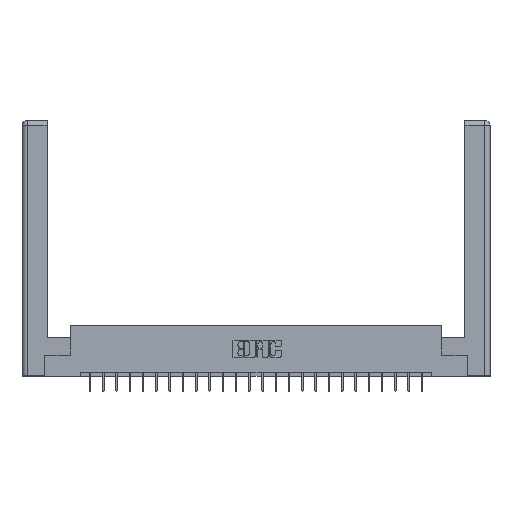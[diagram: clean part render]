
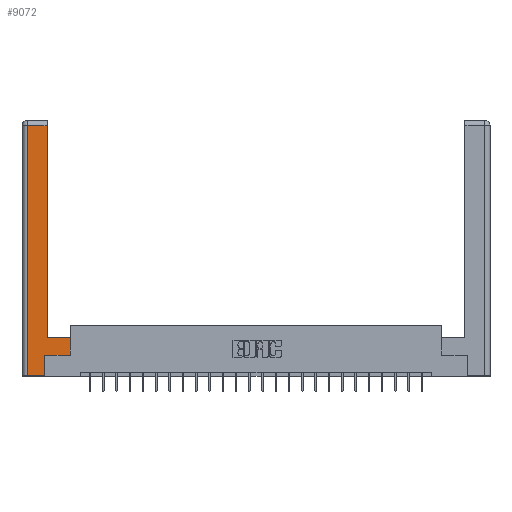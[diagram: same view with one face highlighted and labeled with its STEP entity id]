
A CAD part, top view. The second image highlights one B-rep face of the part: STEP entity #9072.
In plain terms, the highlighted planar face has unit normal (0, 0, 1).
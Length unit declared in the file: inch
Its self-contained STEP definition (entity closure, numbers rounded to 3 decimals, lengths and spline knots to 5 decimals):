
#494 = CARTESIAN_POINT ( 'NONE',  ( 0., 0., 0. ) ) ;
#504 = ORIENTED_EDGE ( 'NONE', *, *, #4105, .T. ) ;
#644 = VERTEX_POINT ( 'NONE', #18237 ) ;
#1146 = CARTESIAN_POINT ( 'NONE',  ( 0.265, 0., 0. ) ) ;
#1230 = VECTOR ( 'NONE', #7607, 39.37008 ) ;
#1911 = VERTEX_POINT ( 'NONE', #3624 ) ;
#1975 = DIRECTION ( 'NONE',  ( 0., 1., 0. ) ) ;
#2231 = CARTESIAN_POINT ( 'NONE',  ( 0.265, 0.245, 0. ) ) ;
#2416 = CARTESIAN_POINT ( 'NONE',  ( 0.295, 2.94, 0. ) ) ;
#2636 = ORIENTED_EDGE ( 'NONE', *, *, #12045, .T. ) ;
#3025 = EDGE_CURVE ( 'NONE', #14537, #15812, #10774, .T. ) ;
#3624 = CARTESIAN_POINT ( 'NONE',  ( 0.565, 0.45, 0. ) ) ;
#4055 = LINE ( 'NONE', #14972, #10418 ) ;
#4105 = EDGE_CURVE ( 'NONE', #8498, #1911, #4055, .T. ) ;
#4262 = ORIENTED_EDGE ( 'NONE', *, *, #11429, .T. ) ;
#4433 = ORIENTED_EDGE ( 'NONE', *, *, #24440, .T. ) ;
#4485 = ORIENTED_EDGE ( 'NONE', *, *, #15095, .T. ) ;
#5100 = CARTESIAN_POINT ( 'NONE',  ( 0.0615, 2.94, 0. ) ) ;
#5492 = AXIS2_PLACEMENT_3D ( 'NONE', #494, #16001, #8128 ) ;
#7195 = EDGE_LOOP ( 'NONE', ( #4262, #15938, #24330, #2636, #11196, #4433, #504, #4485 ) ) ;
#7607 = DIRECTION ( 'NONE',  ( -1., 0., 0. ) ) ;
#7742 = CARTESIAN_POINT ( 'NONE',  ( 0.0615, 2.94, 0. ) ) ;
#7967 = DIRECTION ( 'NONE',  ( -1., 0., 0. ) ) ;
#8015 = VECTOR ( 'NONE', #7967, 39.37008 ) ;
#8128 = DIRECTION ( 'NONE',  ( -1., 0., 0. ) ) ;
#8382 = DIRECTION ( 'NONE',  ( 1., 0., 0. ) ) ;
#8387 = VERTEX_POINT ( 'NONE', #24393 ) ;
#8388 = VECTOR ( 'NONE', #1975, 39.37008 ) ;
#8498 = VERTEX_POINT ( 'NONE', #14652 ) ;
#8891 = LINE ( 'NONE', #11740, #8015 ) ;
#9024 = CARTESIAN_POINT ( 'NONE',  ( 0.0615, 0., 0. ) ) ;
#9072 = ADVANCED_FACE ( 'NONE', ( #9119 ), #12063, .F. ) ;
#9119 = FACE_OUTER_BOUND ( 'NONE', #7195, .T. ) ;
#10418 = VECTOR ( 'NONE', #16655, 39.37008 ) ;
#10774 = LINE ( 'NONE', #16896, #17066 ) ;
#11196 = ORIENTED_EDGE ( 'NONE', *, *, #21120, .T. ) ;
#11429 = EDGE_CURVE ( 'NONE', #12279, #15885, #15606, .T. ) ;
#11740 = CARTESIAN_POINT ( 'NONE',  ( 0.295, 0.45, 0. ) ) ;
#12045 = EDGE_CURVE ( 'NONE', #15812, #8387, #19788, .T. ) ;
#12063 = PLANE ( 'NONE',  #5492 ) ;
#12279 = VERTEX_POINT ( 'NONE', #23125 ) ;
#12524 = DIRECTION ( 'NONE',  ( 1., 0., 0. ) ) ;
#13167 = LINE ( 'NONE', #2231, #8388 ) ;
#14217 = DIRECTION ( 'NONE',  ( 0., 1., 0. ) ) ;
#14537 = VERTEX_POINT ( 'NONE', #5100 ) ;
#14652 = CARTESIAN_POINT ( 'NONE',  ( 0.565, 0.245, 0. ) ) ;
#14972 = CARTESIAN_POINT ( 'NONE',  ( 0.565, 0.45, 0. ) ) ;
#15095 = EDGE_CURVE ( 'NONE', #1911, #12279, #8891, .T. ) ;
#15226 = DIRECTION ( 'NONE',  ( 0., -1., 0. ) ) ;
#15606 = LINE ( 'NONE', #16470, #16206 ) ;
#15812 = VERTEX_POINT ( 'NONE', #9024 ) ;
#15885 = VERTEX_POINT ( 'NONE', #2416 ) ;
#15938 = ORIENTED_EDGE ( 'NONE', *, *, #23942, .T. ) ;
#16001 = DIRECTION ( 'NONE',  ( 0., 0., -1. ) ) ;
#16206 = VECTOR ( 'NONE', #14217, 39.37008 ) ;
#16470 = CARTESIAN_POINT ( 'NONE',  ( 0.295, 3., 0. ) ) ;
#16655 = DIRECTION ( 'NONE',  ( 0., 1., 0. ) ) ;
#16896 = CARTESIAN_POINT ( 'NONE',  ( 0.0615, 0., 0. ) ) ;
#17066 = VECTOR ( 'NONE', #15226, 39.37008 ) ;
#18134 = LINE ( 'NONE', #21750, #22661 ) ;
#18237 = CARTESIAN_POINT ( 'NONE',  ( 0.265, 0.245, 0. ) ) ;
#19788 = LINE ( 'NONE', #1146, #21311 ) ;
#19925 = LINE ( 'NONE', #7742, #1230 ) ;
#21120 = EDGE_CURVE ( 'NONE', #8387, #644, #13167, .T. ) ;
#21311 = VECTOR ( 'NONE', #12524, 39.37008 ) ;
#21750 = CARTESIAN_POINT ( 'NONE',  ( 0.565, 0.245, 0. ) ) ;
#22661 = VECTOR ( 'NONE', #8382, 39.37008 ) ;
#23125 = CARTESIAN_POINT ( 'NONE',  ( 0.295, 0.45, 0. ) ) ;
#23942 = EDGE_CURVE ( 'NONE', #15885, #14537, #19925, .T. ) ;
#24330 = ORIENTED_EDGE ( 'NONE', *, *, #3025, .T. ) ;
#24393 = CARTESIAN_POINT ( 'NONE',  ( 0.265, 0., 0. ) ) ;
#24440 = EDGE_CURVE ( 'NONE', #644, #8498, #18134, .T. ) ;
